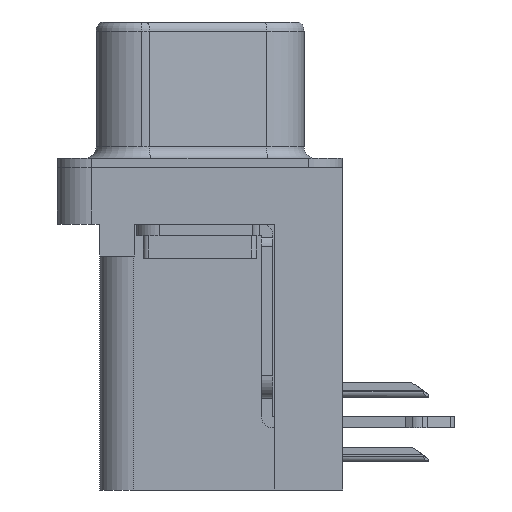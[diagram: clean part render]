
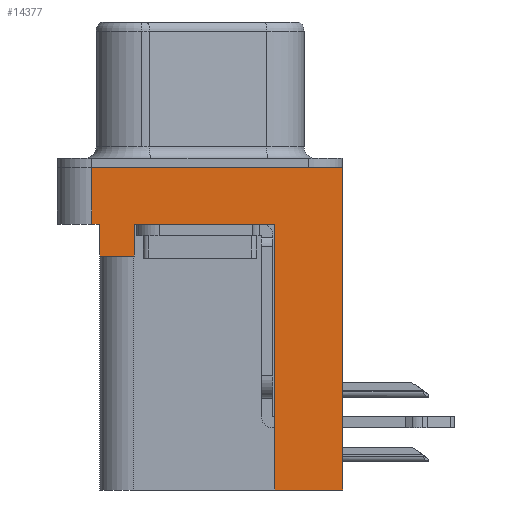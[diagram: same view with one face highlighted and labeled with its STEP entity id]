
A CAD part, left-side view. The second image highlights one B-rep face of the part: STEP entity #14377.
In plain terms, the highlighted planar face has unit normal (-1, 0, 0).
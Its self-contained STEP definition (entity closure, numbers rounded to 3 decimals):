
#533 = DIRECTION ( 'NONE',  ( 0., 0., 1. ) ) ;
#1192 = ORIENTED_EDGE ( 'NONE', *, *, #10175, .F. ) ;
#1219 = PLANE ( 'NONE',  #15450 ) ;
#1445 = CARTESIAN_POINT ( 'NONE',  ( -2.91, -6.275, -2.5 ) ) ;
#1635 = EDGE_CURVE ( 'NONE', #3383, #4664, #16073, .T. ) ;
#1843 = ORIENTED_EDGE ( 'NONE', *, *, #18361, .T. ) ;
#2252 = VECTOR ( 'NONE', #19268, 1000. ) ;
#2312 = LINE ( 'NONE', #10798, #2252 ) ;
#3054 = CARTESIAN_POINT ( 'NONE',  ( -2.91, -3.295, -2.5 ) ) ;
#3371 = VECTOR ( 'NONE', #533, 1000. ) ;
#3383 = VERTEX_POINT ( 'NONE', #9409 ) ;
#4404 = ORIENTED_EDGE ( 'NONE', *, *, #25541, .F. ) ;
#4664 = VERTEX_POINT ( 'NONE', #24100 ) ;
#4835 = CARTESIAN_POINT ( 'NONE',  ( -2.91, -6.275, 0. ) ) ;
#4905 = VECTOR ( 'NONE', #13062, 1000. ) ;
#5388 = CARTESIAN_POINT ( 'NONE',  ( -2.91, -3.295, -14.2 ) ) ;
#5413 = CARTESIAN_POINT ( 'NONE',  ( -2.91, -6.275, -2.5 ) ) ;
#5825 = LINE ( 'NONE', #20543, #9600 ) ;
#6066 = EDGE_CURVE ( 'NONE', #21406, #27193, #10860, .T. ) ;
#6368 = DIRECTION ( 'NONE',  ( 0., 0., 1. ) ) ;
#6458 = CARTESIAN_POINT ( 'NONE',  ( -2.91, -6.275, -2.5 ) ) ;
#6658 = EDGE_CURVE ( 'NONE', #21406, #16958, #24417, .T. ) ;
#6859 = EDGE_CURVE ( 'NONE', #9296, #27193, #5825, .T. ) ;
#7214 = FACE_OUTER_BOUND ( 'NONE', #22026, .T. ) ;
#7744 = LINE ( 'NONE', #26938, #8212 ) ;
#8212 = VECTOR ( 'NONE', #9704, 1000. ) ;
#8305 = CARTESIAN_POINT ( 'NONE',  ( -2.91, 2.895, -3.9 ) ) ;
#9107 = ORIENTED_EDGE ( 'NONE', *, *, #6658, .F. ) ;
#9296 = VERTEX_POINT ( 'NONE', #21238 ) ;
#9409 = CARTESIAN_POINT ( 'NONE',  ( -2.91, -6.275, -14.2 ) ) ;
#9481 = VERTEX_POINT ( 'NONE', #11508 ) ;
#9600 = VECTOR ( 'NONE', #26943, 1000. ) ;
#9702 = ORIENTED_EDGE ( 'NONE', *, *, #6859, .F. ) ;
#9704 = DIRECTION ( 'NONE',  ( 0., 1., 0. ) ) ;
#9819 = EDGE_CURVE ( 'NONE', #23331, #9481, #25385, .T. ) ;
#10090 = DIRECTION ( 'NONE',  ( 0., 0., 1. ) ) ;
#10175 = EDGE_CURVE ( 'NONE', #4664, #26705, #23124, .T. ) ;
#10427 = VECTOR ( 'NONE', #25748, 1000. ) ;
#10798 = CARTESIAN_POINT ( 'NONE',  ( -2.91, -6.275, 0. ) ) ;
#10860 = LINE ( 'NONE', #13212, #12680 ) ;
#11206 = CARTESIAN_POINT ( 'NONE',  ( -2.91, 2.895, -3.9 ) ) ;
#11464 = EDGE_CURVE ( 'NONE', #23331, #9296, #7744, .T. ) ;
#11508 = CARTESIAN_POINT ( 'NONE',  ( -2.91, 2.895, -2.5 ) ) ;
#12009 = LINE ( 'NONE', #1445, #27360 ) ;
#12306 = CARTESIAN_POINT ( 'NONE',  ( -2.91, -3.295, -14.2 ) ) ;
#12680 = VECTOR ( 'NONE', #16979, 1000. ) ;
#13062 = DIRECTION ( 'NONE',  ( 0., 1., 0. ) ) ;
#13212 = CARTESIAN_POINT ( 'NONE',  ( -2.91, -6.275, -2.5 ) ) ;
#13634 = ORIENTED_EDGE ( 'NONE', *, *, #11464, .F. ) ;
#13872 = DIRECTION ( 'NONE',  ( 0., 0., 1. ) ) ;
#14377 = ADVANCED_FACE ( 'NONE', ( #7214 ), #1219, .T. ) ;
#14959 = ORIENTED_EDGE ( 'NONE', *, *, #1635, .F. ) ;
#15450 = AXIS2_PLACEMENT_3D ( 'NONE', #5413, #15955, #13872 ) ;
#15784 = CARTESIAN_POINT ( 'NONE',  ( -2.91, 4.775, -2.5 ) ) ;
#15810 = CARTESIAN_POINT ( 'NONE',  ( -2.91, 4.775, -2.5 ) ) ;
#15955 = DIRECTION ( 'NONE',  ( -1., 0., 0. ) ) ;
#16073 = LINE ( 'NONE', #5388, #4905 ) ;
#16958 = VERTEX_POINT ( 'NONE', #24790 ) ;
#16979 = DIRECTION ( 'NONE',  ( 0., -1., 0. ) ) ;
#17119 = EDGE_CURVE ( 'NONE', #9481, #26705, #21295, .T. ) ;
#18114 = VECTOR ( 'NONE', #6368, 1000. ) ;
#18361 = EDGE_CURVE ( 'NONE', #3383, #21271, #12009, .T. ) ;
#18594 = VECTOR ( 'NONE', #10090, 1000. ) ;
#19268 = DIRECTION ( 'NONE',  ( 0., -1., 0. ) ) ;
#20543 = CARTESIAN_POINT ( 'NONE',  ( -2.91, 4.425, -3.9 ) ) ;
#21238 = CARTESIAN_POINT ( 'NONE',  ( -2.91, 4.425, -3.9 ) ) ;
#21271 = VERTEX_POINT ( 'NONE', #4835 ) ;
#21295 = LINE ( 'NONE', #6458, #10427 ) ;
#21406 = VERTEX_POINT ( 'NONE', #15784 ) ;
#22026 = EDGE_LOOP ( 'NONE', ( #4404, #9107, #25014, #9702, #13634, #25260, #24849, #1192, #14959, #1843 ) ) ;
#23124 = LINE ( 'NONE', #12306, #18594 ) ;
#23331 = VERTEX_POINT ( 'NONE', #11206 ) ;
#24025 = CARTESIAN_POINT ( 'NONE',  ( -2.91, 4.425, -2.5 ) ) ;
#24100 = CARTESIAN_POINT ( 'NONE',  ( -2.91, -3.295, -14.2 ) ) ;
#24417 = LINE ( 'NONE', #15810, #3371 ) ;
#24790 = CARTESIAN_POINT ( 'NONE',  ( -2.91, 4.775, 0. ) ) ;
#24794 = DIRECTION ( 'NONE',  ( 0., 0., 1. ) ) ;
#24849 = ORIENTED_EDGE ( 'NONE', *, *, #17119, .T. ) ;
#25014 = ORIENTED_EDGE ( 'NONE', *, *, #6066, .T. ) ;
#25260 = ORIENTED_EDGE ( 'NONE', *, *, #9819, .T. ) ;
#25385 = LINE ( 'NONE', #8305, #18114 ) ;
#25541 = EDGE_CURVE ( 'NONE', #16958, #21271, #2312, .T. ) ;
#25748 = DIRECTION ( 'NONE',  ( 0., -1., 0. ) ) ;
#26705 = VERTEX_POINT ( 'NONE', #3054 ) ;
#26938 = CARTESIAN_POINT ( 'NONE',  ( -2.91, 4.425, -3.9 ) ) ;
#26943 = DIRECTION ( 'NONE',  ( 0., 0., 1. ) ) ;
#27193 = VERTEX_POINT ( 'NONE', #24025 ) ;
#27360 = VECTOR ( 'NONE', #24794, 1000. ) ;
